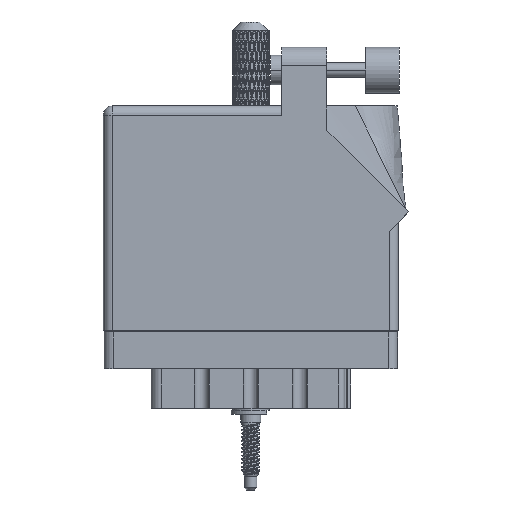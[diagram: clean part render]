
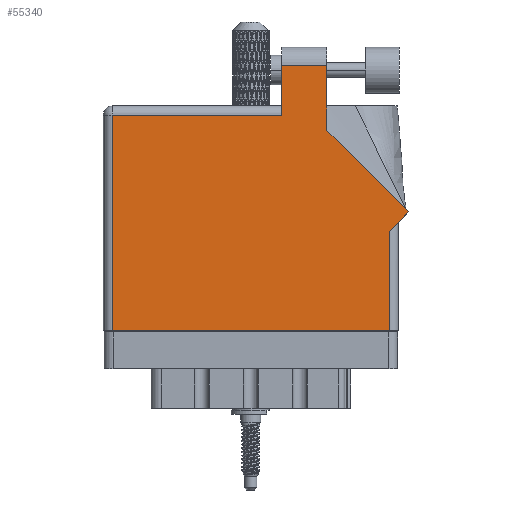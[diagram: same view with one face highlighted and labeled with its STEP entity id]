
A CAD part, front view. The second image highlights one B-rep face of the part: STEP entity #55340.
In plain terms, the highlighted face is planar.
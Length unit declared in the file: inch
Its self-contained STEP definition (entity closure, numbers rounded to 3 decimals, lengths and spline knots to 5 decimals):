
#968 = VECTOR ( 'NONE', #29777, 39.37008 ) ;
#3100 = CARTESIAN_POINT ( 'NONE',  ( 1.217, 1.468, 0. ) ) ;
#4134 = VERTEX_POINT ( 'NONE', #104893 ) ;
#6528 = CARTESIAN_POINT ( 'NONE',  ( 1.524, 1.36442, 0. ) ) ;
#7725 = LINE ( 'NONE', #6528, #77406 ) ;
#8076 = ORIENTED_EDGE ( 'NONE', *, *, #79589, .T. ) ;
#8217 = CARTESIAN_POINT ( 'NONE',  ( 0.062, 0., 0. ) ) ;
#8776 = VECTOR ( 'NONE', #26453, 39.37008 ) ;
#12294 = DIRECTION ( 'NONE',  ( 0., -1., 0. ) ) ;
#12482 = CARTESIAN_POINT ( 'NONE',  ( 1.948, 0.737, 0. ) ) ;
#14031 = EDGE_CURVE ( 'NONE', #84460, #39956, #29381, .T. ) ;
#17854 = ORIENTED_EDGE ( 'NONE', *, *, #67951, .T. ) ;
#21309 = DIRECTION ( 'NONE',  ( -0.707, 0.707, 0. ) ) ;
#21594 = EDGE_LOOP ( 'NONE', ( #90279, #31658, #75902, #106659, #17854, #104721, #66550, #107084, #8076 ) ) ;
#22051 = EDGE_CURVE ( 'NONE', #4134, #43006, #81696, .T. ) ;
#24188 = VECTOR ( 'NONE', #50304, 39.37008 ) ;
#24954 = VECTOR ( 'NONE', #68666, 39.37008 ) ;
#25387 = PLANE ( 'NONE',  #101914 ) ;
#25582 = LINE ( 'NONE', #83395, #8776 ) ;
#26453 = DIRECTION ( 'NONE',  ( 0.707, 0.707, 0. ) ) ;
#27728 = CARTESIAN_POINT ( 'NONE',  ( 2.08071, 0.80771, 0. ) ) ;
#29381 = LINE ( 'NONE', #91053, #24188 ) ;
#29777 = DIRECTION ( 'NONE',  ( 0., -1., 0. ) ) ;
#31435 = DIRECTION ( 'NONE',  ( 0., 1., 0. ) ) ;
#31658 = ORIENTED_EDGE ( 'NONE', *, *, #14031, .T. ) ;
#31669 = VECTOR ( 'NONE', #21309, 39.37008 ) ;
#32268 = VECTOR ( 'NONE', #78376, 39.37008 ) ;
#33686 = DIRECTION ( 'NONE',  ( 0., 0., -1. ) ) ;
#34611 = VERTEX_POINT ( 'NONE', #3100 ) ;
#37897 = CARTESIAN_POINT ( 'NONE',  ( 0.062, 0., 0. ) ) ;
#39956 = VERTEX_POINT ( 'NONE', #66610 ) ;
#40610 = LINE ( 'NONE', #70288, #31669 ) ;
#43006 = VERTEX_POINT ( 'NONE', #64243 ) ;
#47678 = VERTEX_POINT ( 'NONE', #79013 ) ;
#47917 = EDGE_CURVE ( 'NONE', #73282, #84460, #7725, .T. ) ;
#48300 = CARTESIAN_POINT ( 'NONE',  ( 1.524, 1.36442, 0. ) ) ;
#50304 = DIRECTION ( 'NONE',  ( -1., 0., 0. ) ) ;
#53824 = VECTOR ( 'NONE', #12294, 39.37008 ) ;
#55340 = ADVANCED_FACE ( 'NONE', ( #60462 ), #25387, .F. ) ;
#56730 = EDGE_CURVE ( 'NONE', #34611, #47678, #91449, .T. ) ;
#57194 = EDGE_CURVE ( 'NONE', #43006, #94012, #25582, .T. ) ;
#60462 = FACE_OUTER_BOUND ( 'NONE', #21594, .T. ) ;
#61458 = CARTESIAN_POINT ( 'NONE',  ( 1.217, 1.53, 0. ) ) ;
#62828 = CARTESIAN_POINT ( 'NONE',  ( 0., 0., 0. ) ) ;
#64243 = CARTESIAN_POINT ( 'NONE',  ( 1.948, 0.675, 0. ) ) ;
#65663 = VERTEX_POINT ( 'NONE', #8217 ) ;
#66550 = ORIENTED_EDGE ( 'NONE', *, *, #22051, .T. ) ;
#66610 = CARTESIAN_POINT ( 'NONE',  ( 1.217, 1.805, 0. ) ) ;
#67951 = EDGE_CURVE ( 'NONE', #47678, #65663, #89925, .T. ) ;
#68666 = DIRECTION ( 'NONE',  ( 0., 1., 0. ) ) ;
#70288 = CARTESIAN_POINT ( 'NONE',  ( 2.08071, 0.80771, 0. ) ) ;
#73282 = VERTEX_POINT ( 'NONE', #48300 ) ;
#75902 = ORIENTED_EDGE ( 'NONE', *, *, #102033, .T. ) ;
#77406 = VECTOR ( 'NONE', #31435, 39.37008 ) ;
#78376 = DIRECTION ( 'NONE',  ( 1., 0., 0. ) ) ;
#78379 = LINE ( 'NONE', #61458, #968 ) ;
#79013 = CARTESIAN_POINT ( 'NONE',  ( 0.062, 1.468, 0. ) ) ;
#79589 = EDGE_CURVE ( 'NONE', #94012, #73282, #40610, .T. ) ;
#80354 = DIRECTION ( 'NONE',  ( -1., 0., 0. ) ) ;
#81696 = LINE ( 'NONE', #12482, #24954 ) ;
#83030 = CARTESIAN_POINT ( 'NONE',  ( 0., 1.53, 0. ) ) ;
#83395 = CARTESIAN_POINT ( 'NONE',  ( 2.01, 0.737, 0. ) ) ;
#84460 = VERTEX_POINT ( 'NONE', #95218 ) ;
#86299 = VECTOR ( 'NONE', #80354, 39.37008 ) ;
#89925 = LINE ( 'NONE', #37897, #53824 ) ;
#90279 = ORIENTED_EDGE ( 'NONE', *, *, #47917, .T. ) ;
#91053 = CARTESIAN_POINT ( 'NONE',  ( 1.217, 1.805, 0. ) ) ;
#91333 = DIRECTION ( 'NONE',  ( -1., 0., 0. ) ) ;
#91449 = LINE ( 'NONE', #104637, #86299 ) ;
#94012 = VERTEX_POINT ( 'NONE', #27728 ) ;
#95218 = CARTESIAN_POINT ( 'NONE',  ( 1.524, 1.805, 0. ) ) ;
#99566 = EDGE_CURVE ( 'NONE', #65663, #4134, #107104, .T. ) ;
#101914 = AXIS2_PLACEMENT_3D ( 'NONE', #83030, #33686, #91333 ) ;
#102033 = EDGE_CURVE ( 'NONE', #39956, #34611, #78379, .T. ) ;
#104637 = CARTESIAN_POINT ( 'NONE',  ( 0., 1.468, 0. ) ) ;
#104721 = ORIENTED_EDGE ( 'NONE', *, *, #99566, .T. ) ;
#104893 = CARTESIAN_POINT ( 'NONE',  ( 1.948, 0., 0. ) ) ;
#106659 = ORIENTED_EDGE ( 'NONE', *, *, #56730, .T. ) ;
#107084 = ORIENTED_EDGE ( 'NONE', *, *, #57194, .T. ) ;
#107104 = LINE ( 'NONE', #62828, #32268 ) ;
